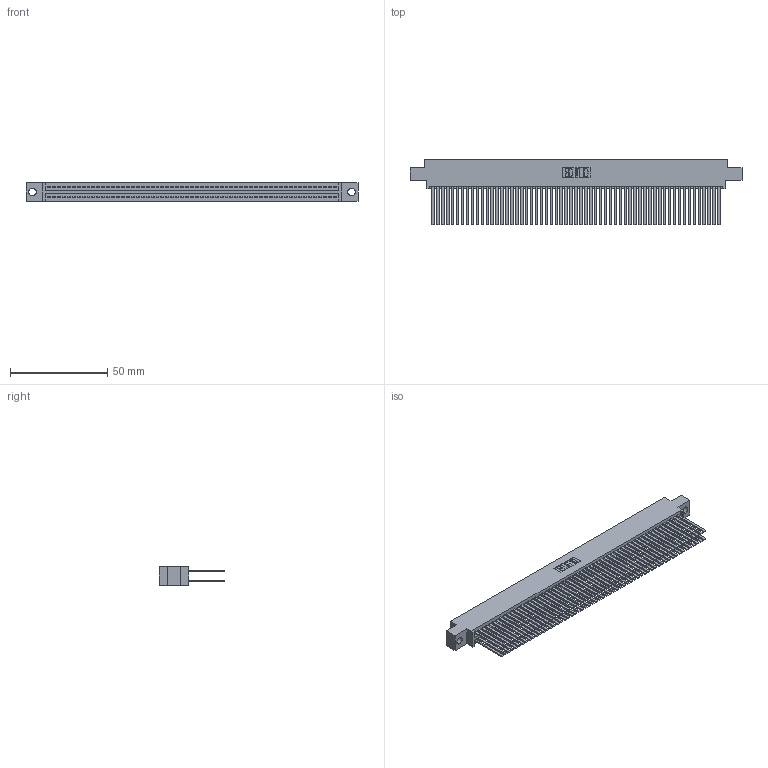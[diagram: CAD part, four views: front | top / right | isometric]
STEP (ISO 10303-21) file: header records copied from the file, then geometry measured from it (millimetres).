
FILE_DESCRIPTION (( 'STEP AP203' ), '1' );
FILE_NAME ('345-118-544-804.STEP', '2018-10-18T22:59:43', ( '' ), ( '' ), 'SwSTEP 2.0', 'SolidWorks 2016', '' );
FILE_SCHEMA (( 'CONFIG_CONTROL_DESIGN' ));
Length unit declared in the file: inch
Products named in the file (3): 345 Part_0.170 Offset - 0.156 Dia-TH; 345-292-001_345-293-144; 345-118-544-804
Assembly tree (119 placements, depth 2):
  345-118-544-804
    345 Part_0.170 Offset - 0.156 Dia-TH
    345-292-001_345-293-144  x118
Bounding box: 171.07 x 33.96 x 9.4 mm (x, y, z)
Volume: 18228.5 mm3; surface area: 32080.9 mm2
Topology: 119 solids, 119 shells, 5322 faces, 15811 edges, 10382 vertices
Faces by surface type: plane 3506, cylinder 1816
Entity records: 43955 total; most frequent: CARTESIAN_POINT 7352, ORIENTED_EDGE 7286, DIRECTION 6459, EDGE_CURVE 3643, VECTOR 3279, LINE 3279, VERTEX_POINT 2426, AXIS2_PLACEMENT_3D 1590
